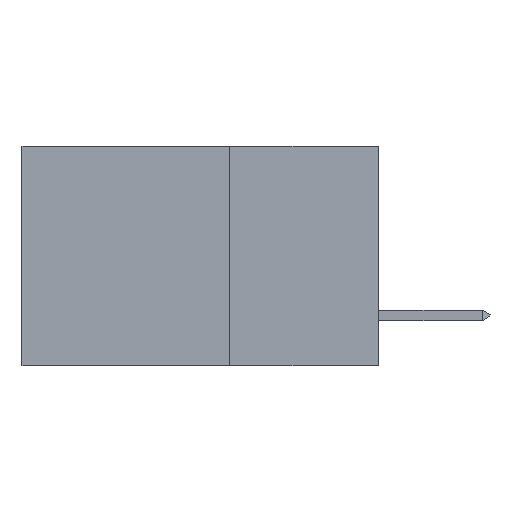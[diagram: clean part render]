
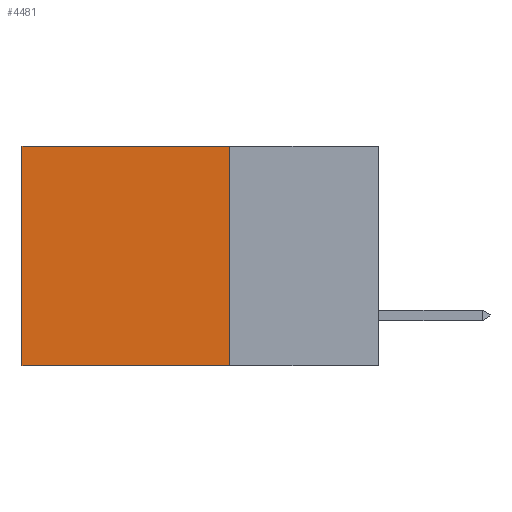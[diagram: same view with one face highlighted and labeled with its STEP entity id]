
A CAD part, left-side view. The second image highlights one B-rep face of the part: STEP entity #4481.
In plain terms, the highlighted planar face has unit normal (-1, 0, 0).
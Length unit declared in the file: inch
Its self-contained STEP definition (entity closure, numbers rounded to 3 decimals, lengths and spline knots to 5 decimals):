
#464 = DIRECTION ( 'NONE',  ( 1., 0., 0. ) ) ;
#640 = ORIENTED_EDGE ( 'NONE', *, *, #10395, .T. ) ;
#918 = CARTESIAN_POINT ( 'NONE',  ( 0.298, 0.6, 0. ) ) ;
#980 = CARTESIAN_POINT ( 'NONE',  ( 0.298, 0.25, 0. ) ) ;
#1108 = EDGE_LOOP ( 'NONE', ( #7739, #8930, #1562, #640 ) ) ;
#1556 = VECTOR ( 'NONE', #9555, 39.37008 ) ;
#1562 = ORIENTED_EDGE ( 'NONE', *, *, #9286, .F. ) ;
#1843 = CARTESIAN_POINT ( 'NONE',  ( 0.298, 0.25, -0.37 ) ) ;
#2153 = CARTESIAN_POINT ( 'NONE',  ( 0.298, 0.6, 0. ) ) ;
#2320 = CARTESIAN_POINT ( 'NONE',  ( 0.298, 0.25, -0.37 ) ) ;
#2455 = CARTESIAN_POINT ( 'NONE',  ( 0.298, 0.25, 0. ) ) ;
#3416 = AXIS2_PLACEMENT_3D ( 'NONE', #4845, #464, #6592 ) ;
#3912 = LINE ( 'NONE', #1843, #1556 ) ;
#4208 = VERTEX_POINT ( 'NONE', #980 ) ;
#4428 = VECTOR ( 'NONE', #5031, 39.37008 ) ;
#4432 = LINE ( 'NONE', #2153, #10831 ) ;
#4481 = ADVANCED_FACE ( 'NONE', ( #5635 ), #9092, .F. ) ;
#4845 = CARTESIAN_POINT ( 'NONE',  ( 0.298, 0.25, 0. ) ) ;
#4853 = EDGE_CURVE ( 'NONE', #7200, #6624, #3912, .T. ) ;
#5031 = DIRECTION ( 'NONE',  ( 0., 1., 0. ) ) ;
#5635 = FACE_OUTER_BOUND ( 'NONE', #1108, .T. ) ;
#5697 = VERTEX_POINT ( 'NONE', #918 ) ;
#5887 = EDGE_CURVE ( 'NONE', #5697, #6624, #4432, .T. ) ;
#6033 = CARTESIAN_POINT ( 'NONE',  ( 0.298, 0.25, 0. ) ) ;
#6592 = DIRECTION ( 'NONE',  ( 0., 0., -1. ) ) ;
#6624 = VERTEX_POINT ( 'NONE', #8404 ) ;
#6724 = LINE ( 'NONE', #2455, #4428 ) ;
#7200 = VERTEX_POINT ( 'NONE', #2320 ) ;
#7350 = DIRECTION ( 'NONE',  ( 0., 0., -1. ) ) ;
#7739 = ORIENTED_EDGE ( 'NONE', *, *, #5887, .T. ) ;
#8029 = VECTOR ( 'NONE', #10977, 39.37008 ) ;
#8404 = CARTESIAN_POINT ( 'NONE',  ( 0.298, 0.6, -0.37 ) ) ;
#8930 = ORIENTED_EDGE ( 'NONE', *, *, #4853, .F. ) ;
#9092 = PLANE ( 'NONE',  #3416 ) ;
#9286 = EDGE_CURVE ( 'NONE', #4208, #7200, #9922, .T. ) ;
#9555 = DIRECTION ( 'NONE',  ( 0., 1., 0. ) ) ;
#9922 = LINE ( 'NONE', #6033, #8029 ) ;
#10395 = EDGE_CURVE ( 'NONE', #4208, #5697, #6724, .T. ) ;
#10831 = VECTOR ( 'NONE', #7350, 39.37008 ) ;
#10977 = DIRECTION ( 'NONE',  ( 0., 0., -1. ) ) ;
